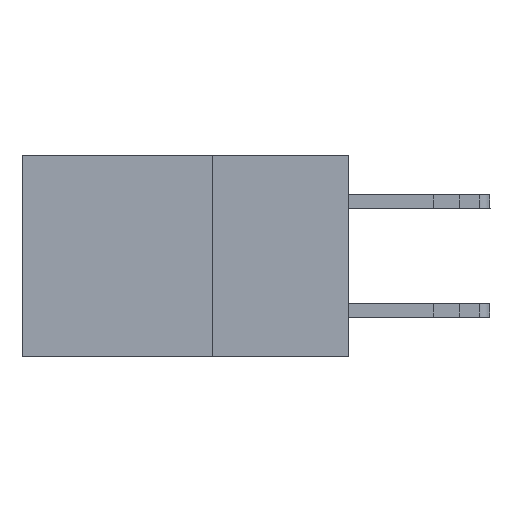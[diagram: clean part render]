
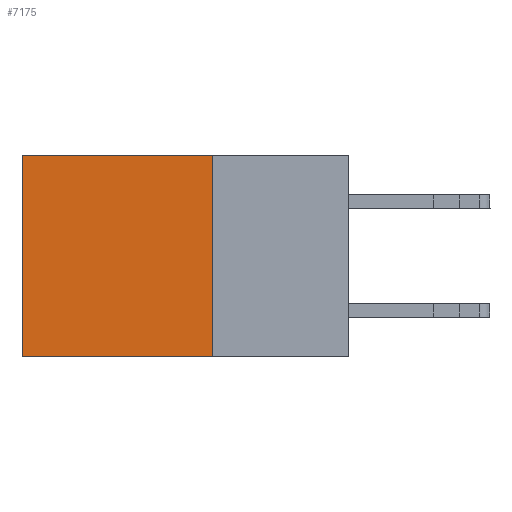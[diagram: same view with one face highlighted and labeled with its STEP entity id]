
A CAD part, left-side view. The second image highlights one B-rep face of the part: STEP entity #7175.
In plain terms, the highlighted planar face has unit normal (-1, 0, 0).
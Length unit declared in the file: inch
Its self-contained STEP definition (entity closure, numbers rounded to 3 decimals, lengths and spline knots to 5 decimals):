
#87 = FACE_OUTER_BOUND ( 'NONE', #8405, .T. ) ;
#719 = EDGE_CURVE ( 'NONE', #9090, #12922, #6424, .T. ) ;
#1806 = PLANE ( 'NONE',  #2640 ) ;
#2458 = VERTEX_POINT ( 'NONE', #5857 ) ;
#2640 = AXIS2_PLACEMENT_3D ( 'NONE', #3265, #10662, #5419 ) ;
#3265 = CARTESIAN_POINT ( 'NONE',  ( 0.298, 0.25, 0. ) ) ;
#3771 = VERTEX_POINT ( 'NONE', #10463 ) ;
#4066 = ORIENTED_EDGE ( 'NONE', *, *, #5621, .T. ) ;
#4435 = CARTESIAN_POINT ( 'NONE',  ( 0.298, 0.25, -0.37 ) ) ;
#4907 = LINE ( 'NONE', #9170, #12371 ) ;
#5419 = DIRECTION ( 'NONE',  ( 0., 0., -1. ) ) ;
#5448 = ORIENTED_EDGE ( 'NONE', *, *, #719, .F. ) ;
#5621 = EDGE_CURVE ( 'NONE', #3771, #2458, #4907, .T. ) ;
#5857 = CARTESIAN_POINT ( 'NONE',  ( 0.298, 0.6, -0.37 ) ) ;
#6284 = DIRECTION ( 'NONE',  ( 0., 0., -1. ) ) ;
#6424 = LINE ( 'NONE', #10553, #9034 ) ;
#6470 = DIRECTION ( 'NONE',  ( 0., 1., 0. ) ) ;
#7175 = ADVANCED_FACE ( 'NONE', ( #87 ), #1806, .F. ) ;
#7394 = LINE ( 'NONE', #9610, #12472 ) ;
#7561 = ORIENTED_EDGE ( 'NONE', *, *, #9790, .T. ) ;
#8318 = ORIENTED_EDGE ( 'NONE', *, *, #9778, .F. ) ;
#8405 = EDGE_LOOP ( 'NONE', ( #4066, #8318, #5448, #7561 ) ) ;
#9034 = VECTOR ( 'NONE', #6284, 39.37008 ) ;
#9090 = VERTEX_POINT ( 'NONE', #12357 ) ;
#9170 = CARTESIAN_POINT ( 'NONE',  ( 0.298, 0.6, 0. ) ) ;
#9307 = DIRECTION ( 'NONE',  ( 0., 0., -1. ) ) ;
#9483 = DIRECTION ( 'NONE',  ( 0., 1., 0. ) ) ;
#9610 = CARTESIAN_POINT ( 'NONE',  ( 0.298, 0.25, 0. ) ) ;
#9778 = EDGE_CURVE ( 'NONE', #12922, #2458, #10663, .T. ) ;
#9790 = EDGE_CURVE ( 'NONE', #9090, #3771, #7394, .T. ) ;
#10463 = CARTESIAN_POINT ( 'NONE',  ( 0.298, 0.6, 0. ) ) ;
#10553 = CARTESIAN_POINT ( 'NONE',  ( 0.298, 0.25, 0. ) ) ;
#10662 = DIRECTION ( 'NONE',  ( 1., 0., 0. ) ) ;
#10663 = LINE ( 'NONE', #12688, #13367 ) ;
#12357 = CARTESIAN_POINT ( 'NONE',  ( 0.298, 0.25, 0. ) ) ;
#12371 = VECTOR ( 'NONE', #9307, 39.37008 ) ;
#12472 = VECTOR ( 'NONE', #6470, 39.37008 ) ;
#12688 = CARTESIAN_POINT ( 'NONE',  ( 0.298, 0.25, -0.37 ) ) ;
#12922 = VERTEX_POINT ( 'NONE', #4435 ) ;
#13367 = VECTOR ( 'NONE', #9483, 39.37008 ) ;
